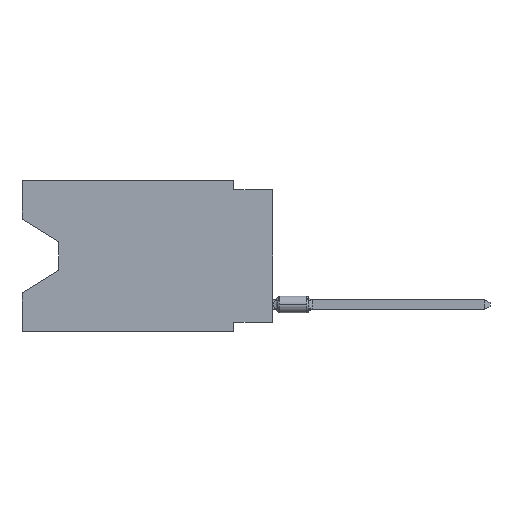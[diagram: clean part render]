
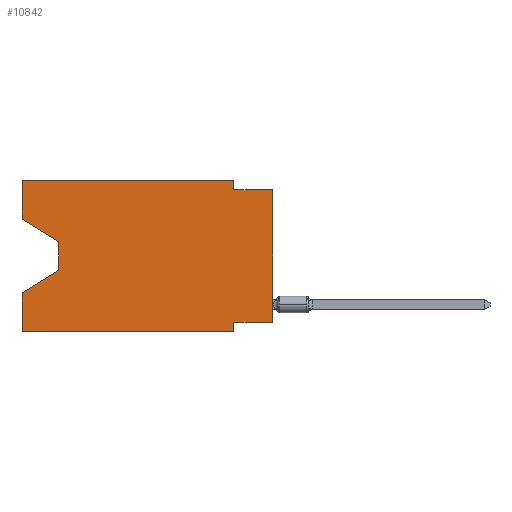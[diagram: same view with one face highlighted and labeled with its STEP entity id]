
A CAD part, left-side view. The second image highlights one B-rep face of the part: STEP entity #10842.
In plain terms, the highlighted planar face has unit normal (-1, 0, 0).
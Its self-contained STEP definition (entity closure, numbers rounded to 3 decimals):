
#462 = LINE ( 'NONE', #12301, #11512 ) ;
#520 = EDGE_CURVE ( 'NONE', #704, #9065, #676, .T. ) ;
#577 = CARTESIAN_POINT ( 'NONE',  ( 0., 16.383, -9.906 ) ) ;
#676 = LINE ( 'NONE', #12673, #13544 ) ;
#696 = EDGE_CURVE ( 'NONE', #10986, #1838, #9237, .T. ) ;
#704 = VERTEX_POINT ( 'NONE', #9313 ) ;
#729 = CARTESIAN_POINT ( 'NONE',  ( 0., 16.383, 0. ) ) ;
#945 = DIRECTION ( 'NONE',  ( 0., 0., 1. ) ) ;
#1182 = EDGE_CURVE ( 'NONE', #10049, #10986, #4051, .T. ) ;
#1235 = EDGE_CURVE ( 'NONE', #14877, #7428, #7080, .T. ) ;
#1322 = AXIS2_PLACEMENT_3D ( 'NONE', #729, #9819, #16220 ) ;
#1564 = CARTESIAN_POINT ( 'NONE',  ( 0., 13.97, -5.893 ) ) ;
#1608 = CARTESIAN_POINT ( 'NONE',  ( 0., 2.54, 0. ) ) ;
#1838 = VERTEX_POINT ( 'NONE', #10272 ) ;
#1901 = CARTESIAN_POINT ( 'NONE',  ( 0., 2.54, -0.635 ) ) ;
#2112 = CARTESIAN_POINT ( 'NONE',  ( 0., 0., -0.635 ) ) ;
#2224 = VERTEX_POINT ( 'NONE', #2112 ) ;
#2355 = ORIENTED_EDGE ( 'NONE', *, *, #9167, .F. ) ;
#2395 = DIRECTION ( 'NONE',  ( 0., 0., 1. ) ) ;
#3146 = DIRECTION ( 'NONE',  ( 0., -1., 0. ) ) ;
#3443 = ORIENTED_EDGE ( 'NONE', *, *, #696, .F. ) ;
#3460 = PLANE ( 'NONE',  #1322 ) ;
#3494 = EDGE_CURVE ( 'NONE', #9065, #9069, #5508, .T. ) ;
#4019 = VERTEX_POINT ( 'NONE', #1901 ) ;
#4051 = LINE ( 'NONE', #14519, #12185 ) ;
#4335 = DIRECTION ( 'NONE',  ( 0., 0., -1. ) ) ;
#4857 = DIRECTION ( 'NONE',  ( 0., -0.855, -0.519 ) ) ;
#5258 = VECTOR ( 'NONE', #2395, 1000. ) ;
#5508 = LINE ( 'NONE', #10840, #13650 ) ;
#5695 = DIRECTION ( 'NONE',  ( 0., 0.855, -0.519 ) ) ;
#5760 = ORIENTED_EDGE ( 'NONE', *, *, #9527, .T. ) ;
#6026 = VECTOR ( 'NONE', #9847, 1000. ) ;
#6445 = VECTOR ( 'NONE', #16797, 1000. ) ;
#6475 = VECTOR ( 'NONE', #3146, 1000. ) ;
#6804 = ORIENTED_EDGE ( 'NONE', *, *, #9743, .T. ) ;
#7080 = LINE ( 'NONE', #7249, #12996 ) ;
#7090 = EDGE_CURVE ( 'NONE', #4019, #2224, #14891, .T. ) ;
#7249 = CARTESIAN_POINT ( 'NONE',  ( 0., 16.383, 0. ) ) ;
#7428 = VERTEX_POINT ( 'NONE', #7683 ) ;
#7440 = CARTESIAN_POINT ( 'NONE',  ( 0., 0., 0. ) ) ;
#7469 = LINE ( 'NONE', #12696, #8924 ) ;
#7683 = CARTESIAN_POINT ( 'NONE',  ( 0., 2.54, 0. ) ) ;
#7750 = CARTESIAN_POINT ( 'NONE',  ( 0., 2.54, -9.271 ) ) ;
#8014 = DIRECTION ( 'NONE',  ( 0., 1., 0. ) ) ;
#8345 = VERTEX_POINT ( 'NONE', #577 ) ;
#8924 = VECTOR ( 'NONE', #945, 1000. ) ;
#9065 = VERTEX_POINT ( 'NONE', #10569 ) ;
#9069 = VERTEX_POINT ( 'NONE', #1564 ) ;
#9167 = EDGE_CURVE ( 'NONE', #704, #14877, #12291, .T. ) ;
#9237 = LINE ( 'NONE', #14715, #11611 ) ;
#9313 = CARTESIAN_POINT ( 'NONE',  ( 0., 16.383, -2.546 ) ) ;
#9373 = CARTESIAN_POINT ( 'NONE',  ( 0., 16.383, 0. ) ) ;
#9527 = EDGE_CURVE ( 'NONE', #10049, #2224, #9586, .T. ) ;
#9586 = LINE ( 'NONE', #7440, #6026 ) ;
#9715 = CARTESIAN_POINT ( 'NONE',  ( 0., 16.383, 0. ) ) ;
#9743 = EDGE_CURVE ( 'NONE', #9069, #16262, #462, .T. ) ;
#9819 = DIRECTION ( 'NONE',  ( 1., 0., 0. ) ) ;
#9847 = DIRECTION ( 'NONE',  ( 0., 0., 1. ) ) ;
#10049 = VERTEX_POINT ( 'NONE', #11220 ) ;
#10272 = CARTESIAN_POINT ( 'NONE',  ( 0., 2.54, -9.906 ) ) ;
#10476 = ORIENTED_EDGE ( 'NONE', *, *, #520, .T. ) ;
#10569 = CARTESIAN_POINT ( 'NONE',  ( 0., 13.97, -4.013 ) ) ;
#10840 = CARTESIAN_POINT ( 'NONE',  ( 0., 13.97, -4.013 ) ) ;
#10842 = ADVANCED_FACE ( 'NONE', ( #12556 ), #3460, .F. ) ;
#10986 = VERTEX_POINT ( 'NONE', #7750 ) ;
#11220 = CARTESIAN_POINT ( 'NONE',  ( 0., 0., -9.271 ) ) ;
#11512 = VECTOR ( 'NONE', #5695, 1000. ) ;
#11611 = VECTOR ( 'NONE', #4335, 1000. ) ;
#12185 = VECTOR ( 'NONE', #8014, 1000. ) ;
#12291 = LINE ( 'NONE', #9715, #5258 ) ;
#12301 = CARTESIAN_POINT ( 'NONE',  ( 0., 13.97, -5.893 ) ) ;
#12327 = CARTESIAN_POINT ( 'NONE',  ( 0., 0., -0.635 ) ) ;
#12556 = FACE_OUTER_BOUND ( 'NONE', #14616, .T. ) ;
#12673 = CARTESIAN_POINT ( 'NONE',  ( 0., 16.383, -2.546 ) ) ;
#12696 = CARTESIAN_POINT ( 'NONE',  ( 0., 16.383, 0. ) ) ;
#12822 = ORIENTED_EDGE ( 'NONE', *, *, #7090, .F. ) ;
#12915 = ORIENTED_EDGE ( 'NONE', *, *, #13175, .F. ) ;
#12996 = VECTOR ( 'NONE', #16381, 1000. ) ;
#13175 = EDGE_CURVE ( 'NONE', #7428, #4019, #13364, .T. ) ;
#13364 = LINE ( 'NONE', #1608, #13985 ) ;
#13544 = VECTOR ( 'NONE', #4857, 1000. ) ;
#13650 = VECTOR ( 'NONE', #16050, 1000. ) ;
#13953 = ORIENTED_EDGE ( 'NONE', *, *, #16471, .T. ) ;
#13985 = VECTOR ( 'NONE', #14387, 1000. ) ;
#14137 = ORIENTED_EDGE ( 'NONE', *, *, #1235, .F. ) ;
#14387 = DIRECTION ( 'NONE',  ( 0., 0., -1. ) ) ;
#14464 = ORIENTED_EDGE ( 'NONE', *, *, #16892, .F. ) ;
#14519 = CARTESIAN_POINT ( 'NONE',  ( 0., 0., -9.271 ) ) ;
#14616 = EDGE_LOOP ( 'NONE', ( #10476, #15573, #6804, #14464, #13953, #3443, #15902, #5760, #12822, #12915, #14137, #2355 ) ) ;
#14715 = CARTESIAN_POINT ( 'NONE',  ( 0., 2.54, -9.906 ) ) ;
#14877 = VERTEX_POINT ( 'NONE', #9373 ) ;
#14891 = LINE ( 'NONE', #12327, #6475 ) ;
#15441 = CARTESIAN_POINT ( 'NONE',  ( 0., 16.383, -9.906 ) ) ;
#15573 = ORIENTED_EDGE ( 'NONE', *, *, #3494, .T. ) ;
#15902 = ORIENTED_EDGE ( 'NONE', *, *, #1182, .F. ) ;
#16049 = CARTESIAN_POINT ( 'NONE',  ( 0., 16.383, -7.36 ) ) ;
#16050 = DIRECTION ( 'NONE',  ( 0., 0., -1. ) ) ;
#16220 = DIRECTION ( 'NONE',  ( 0., 0., -1. ) ) ;
#16262 = VERTEX_POINT ( 'NONE', #16049 ) ;
#16381 = DIRECTION ( 'NONE',  ( 0., -1., 0. ) ) ;
#16471 = EDGE_CURVE ( 'NONE', #8345, #1838, #16716, .T. ) ;
#16716 = LINE ( 'NONE', #15441, #6445 ) ;
#16797 = DIRECTION ( 'NONE',  ( 0., -1., 0. ) ) ;
#16892 = EDGE_CURVE ( 'NONE', #8345, #16262, #7469, .T. ) ;
